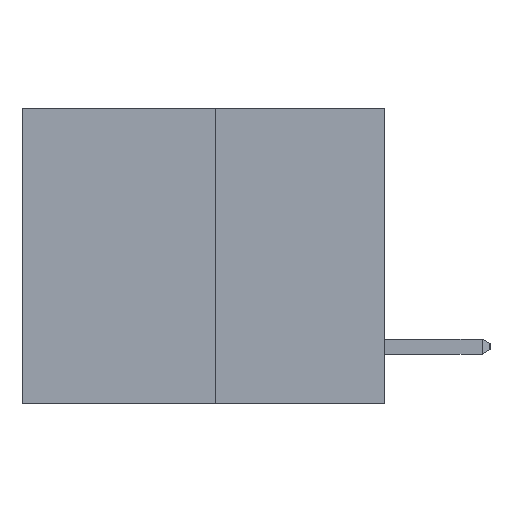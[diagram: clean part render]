
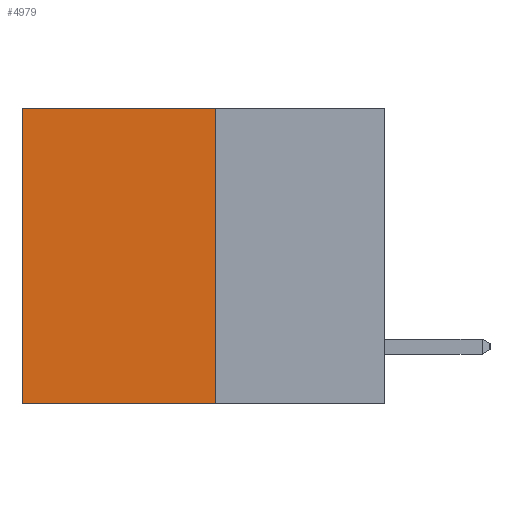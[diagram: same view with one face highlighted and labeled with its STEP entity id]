
A CAD part, left-side view. The second image highlights one B-rep face of the part: STEP entity #4979.
In plain terms, the highlighted planar face has unit normal (-1, 0, 0).
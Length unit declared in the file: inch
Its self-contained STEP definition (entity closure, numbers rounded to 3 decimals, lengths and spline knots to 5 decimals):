
#50 = AXIS2_PLACEMENT_3D ( 'NONE', #12271, #14546, #219 ) ;
#106 = VERTEX_POINT ( 'NONE', #426 ) ;
#206 = CARTESIAN_POINT ( 'NONE',  ( 0.3165, 0.28, -0.49 ) ) ;
#219 = DIRECTION ( 'NONE',  ( 0., 0., -1. ) ) ;
#426 = CARTESIAN_POINT ( 'NONE',  ( 0.3165, 0.6, -0.49 ) ) ;
#465 = CARTESIAN_POINT ( 'NONE',  ( 0.3165, 0.28, -0.49 ) ) ;
#570 = DIRECTION ( 'NONE',  ( 0., 0., -1. ) ) ;
#917 = ORIENTED_EDGE ( 'NONE', *, *, #9851, .F. ) ;
#1137 = VECTOR ( 'NONE', #5371, 39.37008 ) ;
#1386 = ORIENTED_EDGE ( 'NONE', *, *, #8717, .T. ) ;
#1572 = DIRECTION ( 'NONE',  ( 0., 0., -1. ) ) ;
#1660 = DIRECTION ( 'NONE',  ( 0., 1., 0. ) ) ;
#2014 = EDGE_CURVE ( 'NONE', #9430, #5665, #9186, .T. ) ;
#4261 = VECTOR ( 'NONE', #570, 39.37008 ) ;
#4410 = LINE ( 'NONE', #465, #4974 ) ;
#4974 = VECTOR ( 'NONE', #1660, 39.37008 ) ;
#4979 = ADVANCED_FACE ( 'NONE', ( #14761 ), #10894, .F. ) ;
#5371 = DIRECTION ( 'NONE',  ( 0., 1., 0. ) ) ;
#5665 = VERTEX_POINT ( 'NONE', #10981 ) ;
#6094 = VERTEX_POINT ( 'NONE', #10917 ) ;
#7462 = LINE ( 'NONE', #12627, #4261 ) ;
#8349 = CARTESIAN_POINT ( 'NONE',  ( 0.3165, 0.28, 0. ) ) ;
#8717 = EDGE_CURVE ( 'NONE', #6094, #106, #7462, .T. ) ;
#8843 = CARTESIAN_POINT ( 'NONE',  ( 0.3165, 0.28, 0. ) ) ;
#9186 = LINE ( 'NONE', #206, #11847 ) ;
#9430 = VERTEX_POINT ( 'NONE', #8349 ) ;
#9555 = EDGE_LOOP ( 'NONE', ( #1386, #917, #10209, #10748 ) ) ;
#9851 = EDGE_CURVE ( 'NONE', #5665, #106, #4410, .T. ) ;
#9938 = LINE ( 'NONE', #8843, #1137 ) ;
#10209 = ORIENTED_EDGE ( 'NONE', *, *, #2014, .F. ) ;
#10748 = ORIENTED_EDGE ( 'NONE', *, *, #12228, .T. ) ;
#10894 = PLANE ( 'NONE',  #50 ) ;
#10917 = CARTESIAN_POINT ( 'NONE',  ( 0.3165, 0.6, 0. ) ) ;
#10981 = CARTESIAN_POINT ( 'NONE',  ( 0.3165, 0.28, -0.49 ) ) ;
#11847 = VECTOR ( 'NONE', #1572, 39.37008 ) ;
#12228 = EDGE_CURVE ( 'NONE', #9430, #6094, #9938, .T. ) ;
#12271 = CARTESIAN_POINT ( 'NONE',  ( 0.3165, 0.28, -0.49 ) ) ;
#12627 = CARTESIAN_POINT ( 'NONE',  ( 0.3165, 0.6, -0.49 ) ) ;
#14546 = DIRECTION ( 'NONE',  ( 1., 0., 0. ) ) ;
#14761 = FACE_OUTER_BOUND ( 'NONE', #9555, .T. ) ;
